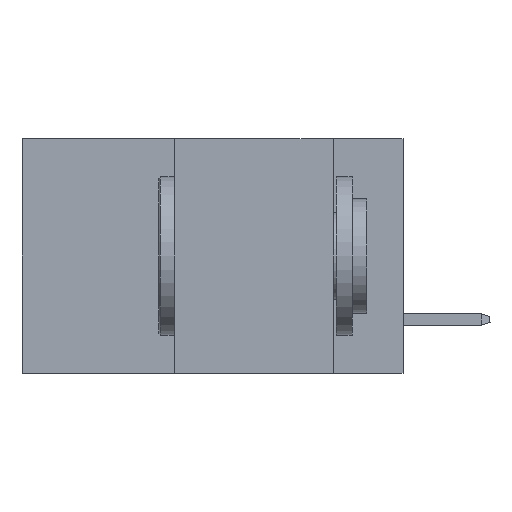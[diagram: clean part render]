
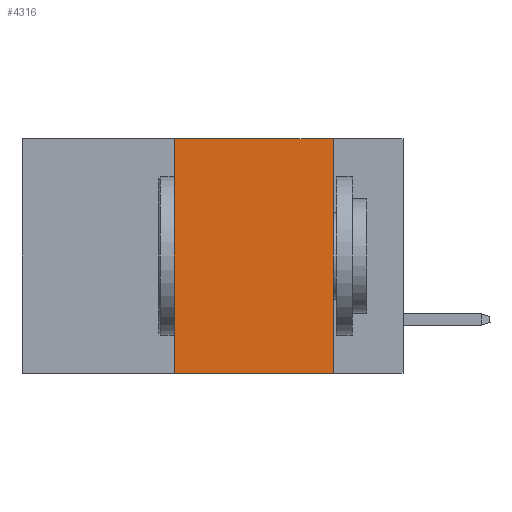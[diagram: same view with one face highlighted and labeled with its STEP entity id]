
A CAD part, left-side view. The second image highlights one B-rep face of the part: STEP entity #4316.
In plain terms, the highlighted planar face has unit normal (-1, 0, 0).
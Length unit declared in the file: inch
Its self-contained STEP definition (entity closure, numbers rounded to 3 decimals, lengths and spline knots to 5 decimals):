
#325 = VERTEX_POINT ( 'NONE', #1221 ) ;
#1116 = CARTESIAN_POINT ( 'NONE',  ( 0., 0.36, -0.37 ) ) ;
#1221 = CARTESIAN_POINT ( 'NONE',  ( 0., 0.11, 0. ) ) ;
#2585 = LINE ( 'NONE', #22549, #18747 ) ;
#4170 = VECTOR ( 'NONE', #10015, 39.37008 ) ;
#4316 = ADVANCED_FACE ( 'NONE', ( #17420 ), #6834, .F. ) ;
#4548 = DIRECTION ( 'NONE',  ( 0., 0., 1. ) ) ;
#5514 = CARTESIAN_POINT ( 'NONE',  ( 0., 0.11, 0. ) ) ;
#6453 = ORIENTED_EDGE ( 'NONE', *, *, #17228, .F. ) ;
#6834 = PLANE ( 'NONE',  #17416 ) ;
#7343 = EDGE_CURVE ( 'NONE', #10282, #8474, #2585, .T. ) ;
#7851 = EDGE_LOOP ( 'NONE', ( #6453, #23087, #9809, #21260 ) ) ;
#8263 = DIRECTION ( 'NONE',  ( 0., -1., 0. ) ) ;
#8474 = VERTEX_POINT ( 'NONE', #17411 ) ;
#9664 = CARTESIAN_POINT ( 'NONE',  ( 0., 0.6, 0. ) ) ;
#9809 = ORIENTED_EDGE ( 'NONE', *, *, #7343, .F. ) ;
#10011 = DIRECTION ( 'NONE',  ( 1., 0., 0. ) ) ;
#10015 = DIRECTION ( 'NONE',  ( 0., -1., 0. ) ) ;
#10282 = VERTEX_POINT ( 'NONE', #1116 ) ;
#10983 = VECTOR ( 'NONE', #18531, 39.37008 ) ;
#11269 = CARTESIAN_POINT ( 'NONE',  ( 0., 0.11, -0.37 ) ) ;
#12951 = EDGE_CURVE ( 'NONE', #10282, #22426, #15293, .T. ) ;
#13660 = CARTESIAN_POINT ( 'NONE',  ( 0., 0.6, -0.37 ) ) ;
#14426 = VECTOR ( 'NONE', #8263, 39.37008 ) ;
#14754 = LINE ( 'NONE', #5514, #10983 ) ;
#15293 = LINE ( 'NONE', #13660, #4170 ) ;
#17228 = EDGE_CURVE ( 'NONE', #325, #22426, #14754, .T. ) ;
#17411 = CARTESIAN_POINT ( 'NONE',  ( 0., 0.36, 0. ) ) ;
#17416 = AXIS2_PLACEMENT_3D ( 'NONE', #19054, #10011, #17540 ) ;
#17420 = FACE_OUTER_BOUND ( 'NONE', #7851, .T. ) ;
#17540 = DIRECTION ( 'NONE',  ( 0., 0., -1. ) ) ;
#18531 = DIRECTION ( 'NONE',  ( 0., 0., -1. ) ) ;
#18747 = VECTOR ( 'NONE', #4548, 39.37008 ) ;
#18999 = EDGE_CURVE ( 'NONE', #8474, #325, #20487, .T. ) ;
#19054 = CARTESIAN_POINT ( 'NONE',  ( 0., 0.6, 0. ) ) ;
#20487 = LINE ( 'NONE', #9664, #14426 ) ;
#21260 = ORIENTED_EDGE ( 'NONE', *, *, #12951, .T. ) ;
#22426 = VERTEX_POINT ( 'NONE', #11269 ) ;
#22549 = CARTESIAN_POINT ( 'NONE',  ( 0., 0.36, 0. ) ) ;
#23087 = ORIENTED_EDGE ( 'NONE', *, *, #18999, .F. ) ;
